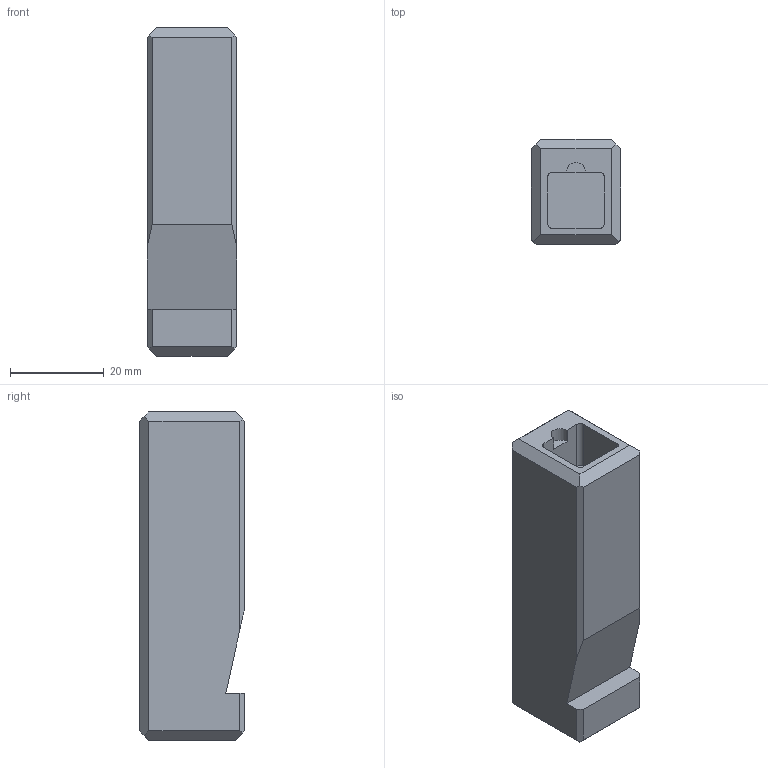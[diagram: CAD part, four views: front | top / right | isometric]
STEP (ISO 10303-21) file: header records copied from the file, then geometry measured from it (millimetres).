
FILE_DESCRIPTION((''),'2;1');
FILE_NAME('PM522Striker2.stp','2015-10-01T18:16:15',('JamesRPatrick'),(''),'Autodesk Inventor 2012','Autodesk Inventor 2012','');
FILE_SCHEMA(('AUTOMOTIVE_DESIGN { 1 0 10303 214 1 1 1 1 }'));
Length unit declared in the file: millimetre
Products named in the file (1): PM522Striker2
Bounding box: 19 x 22.4 x 70 mm (x, y, z)
Volume: 16735.6 mm3; surface area: 8906.9 mm2
Topology: 1 solids, 1 shells, 76 faces, 196 edges, 122 vertices
Faces by surface type: plane 41, cylinder 23, torus 6, sphere 6
Entity records: 2276 total; most frequent: CARTESIAN_POINT 405, DIRECTION 392, ORIENTED_EDGE 380, EDGE_CURVE 190, VECTOR 134, LINE 134, AXIS2_PLACEMENT_3D 129, VERTEX_POINT 118
